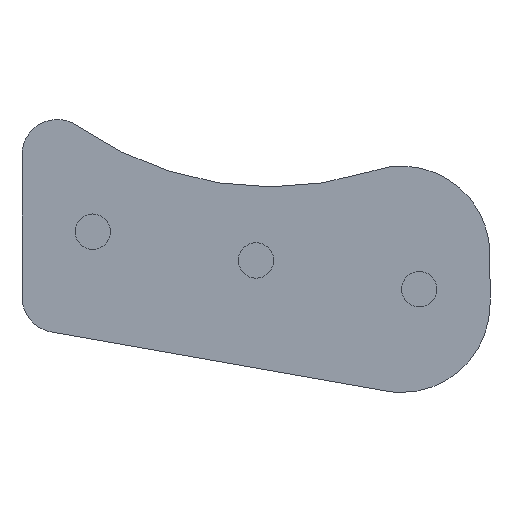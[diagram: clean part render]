
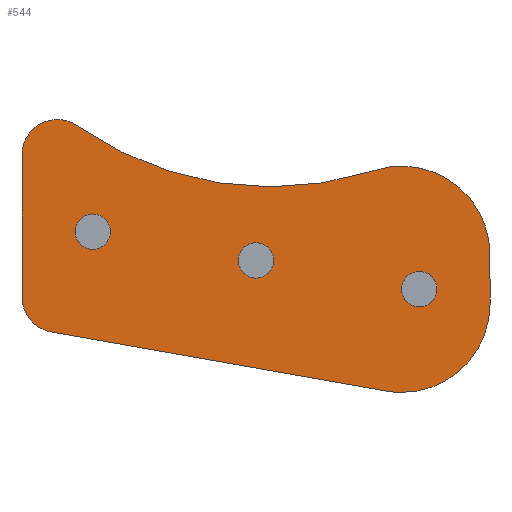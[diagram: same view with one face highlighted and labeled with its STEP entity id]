
A CAD part, left-side view. The second image highlights one B-rep face of the part: STEP entity #544.
In plain terms, the highlighted planar face has unit normal (-1, 0, 0).
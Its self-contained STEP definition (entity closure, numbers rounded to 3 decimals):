
#14 = FACE_BOUND ( 'NONE', #4866, .T. ) ;
#60 = DIRECTION ( 'NONE',  ( 0., 0., -1. ) ) ;
#68 = EDGE_CURVE ( 'NONE', #3412, #212, #5007, .T. ) ;
#90 = CARTESIAN_POINT ( 'NONE',  ( 5., 16.002, -34.415 ) ) ;
#95 = AXIS2_PLACEMENT_3D ( 'NONE', #5192, #797, #5929 ) ;
#101 = DIRECTION ( 'NONE',  ( 0., 0., -1. ) ) ;
#212 = VERTEX_POINT ( 'NONE', #5666 ) ;
#221 = ORIENTED_EDGE ( 'NONE', *, *, #2972, .F. ) ;
#262 = CIRCLE ( 'NONE', #8717, 2.5 ) ;
#370 = ORIENTED_EDGE ( 'NONE', *, *, #1167, .T. ) ;
#393 = DIRECTION ( 'NONE',  ( 1., 0., 0. ) ) ;
#544 = ADVANCED_FACE ( 'NONE', ( #14, #2244, #2038, #2032 ), #2638, .T. ) ;
#551 = CARTESIAN_POINT ( 'NONE',  ( 5., 22.266, -17.584 ) ) ;
#581 = CARTESIAN_POINT ( 'NONE',  ( 5., 8.973, -50.886 ) ) ;
#628 = ORIENTED_EDGE ( 'NONE', *, *, #5931, .T. ) ;
#797 = DIRECTION ( 'NONE',  ( 1., 0., 0. ) ) ;
#824 = DIRECTION ( 'NONE',  ( 0., 0., -1. ) ) ;
#1092 = DIRECTION ( 'NONE',  ( 1., 0., 0. ) ) ;
#1150 = CARTESIAN_POINT ( 'NONE',  ( 5., 16.002, -34.415 ) ) ;
#1167 = EDGE_CURVE ( 'NONE', #2639, #3178, #8629, .T. ) ;
#1358 = CARTESIAN_POINT ( 'NONE',  ( 5., 39.105, -32.842 ) ) ;
#1359 = ORIENTED_EDGE ( 'NONE', *, *, #4983, .F. ) ;
#1401 = VERTEX_POINT ( 'NONE', #3144 ) ;
#1427 = CARTESIAN_POINT ( 'NONE',  ( 5., 16.002, -36.915 ) ) ;
#1443 = ORIENTED_EDGE ( 'NONE', *, *, #1815, .T. ) ;
#1459 = DIRECTION ( 'NONE',  ( 1., 0., 0. ) ) ;
#1531 = VERTEX_POINT ( 'NONE', #3245 ) ;
#1760 = VERTEX_POINT ( 'NONE', #7025 ) ;
#1770 = CARTESIAN_POINT ( 'NONE',  ( 5., 18.502, -36.513 ) ) ;
#1815 = EDGE_CURVE ( 'NONE', #8093, #1892, #6474, .T. ) ;
#1860 = AXIS2_PLACEMENT_3D ( 'NONE', #5502, #1092, #6226 ) ;
#1892 = VERTEX_POINT ( 'NONE', #8812 ) ;
#1895 = DIRECTION ( 'NONE',  ( 0., 0., -1. ) ) ;
#2032 = FACE_OUTER_BOUND ( 'NONE', #8534, .T. ) ;
#2038 = FACE_BOUND ( 'NONE', #4695, .T. ) ;
#2117 = EDGE_CURVE ( 'NONE', #1531, #5927, #5447, .T. ) ;
#2120 = CIRCLE ( 'NONE', #95, 12.5 ) ;
#2172 = CARTESIAN_POINT ( 'NONE',  ( 5., 62.208, -28.768 ) ) ;
#2195 = EDGE_CURVE ( 'NONE', #1760, #6677, #4984, .T. ) ;
#2219 = LINE ( 'NONE', #4430, #2228 ) ;
#2228 = VECTOR ( 'NONE', #60, 1000. ) ;
#2244 = FACE_BOUND ( 'NONE', #3568, .T. ) ;
#2348 = AXIS2_PLACEMENT_3D ( 'NONE', #2391, #7439, #3117 ) ;
#2357 = CARTESIAN_POINT ( 'NONE',  ( 5., 18.502, -29.504 ) ) ;
#2391 = CARTESIAN_POINT ( 'NONE',  ( 5., 62.208, -26.268 ) ) ;
#2432 = EDGE_CURVE ( 'NONE', #4355, #1401, #3818, .T. ) ;
#2502 = DIRECTION ( 'NONE',  ( 0., 0., -1. ) ) ;
#2520 = ORIENTED_EDGE ( 'NONE', *, *, #2117, .T. ) ;
#2608 = ORIENTED_EDGE ( 'NONE', *, *, #68, .F. ) ;
#2638 = PLANE ( 'NONE',  #4228 ) ;
#2639 = VERTEX_POINT ( 'NONE', #5607 ) ;
#2671 = AXIS2_PLACEMENT_3D ( 'NONE', #5453, #1459, #4809 ) ;
#2704 = CARTESIAN_POINT ( 'NONE',  ( 5., 72.208, -15.407 ) ) ;
#2972 = EDGE_CURVE ( 'NONE', #4893, #5985, #2120, .T. ) ;
#3070 = AXIS2_PLACEMENT_3D ( 'NONE', #2357, #7401, #3079 ) ;
#3079 = DIRECTION ( 'NONE',  ( 0., 0., -1. ) ) ;
#3117 = DIRECTION ( 'NONE',  ( 0., 0., -1. ) ) ;
#3144 = CARTESIAN_POINT ( 'NONE',  ( 5., 6.002, -29.504 ) ) ;
#3178 = VERTEX_POINT ( 'NONE', #4520 ) ;
#3245 = CARTESIAN_POINT ( 'NONE',  ( 5., 16.002, -31.915 ) ) ;
#3342 = CARTESIAN_POINT ( 'NONE',  ( 5., 67.208, -35.541 ) ) ;
#3412 = VERTEX_POINT ( 'NONE', #8538 ) ;
#3444 = ORIENTED_EDGE ( 'NONE', *, *, #6522, .T. ) ;
#3568 = EDGE_LOOP ( 'NONE', ( #7085, #2520 ) ) ;
#3595 = DIRECTION ( 'NONE',  ( 1., 0., 0. ) ) ;
#3625 = CARTESIAN_POINT ( 'NONE',  ( 5., 18.502, -49.013 ) ) ;
#3626 = ORIENTED_EDGE ( 'NONE', *, *, #2195, .F. ) ;
#3627 = VECTOR ( 'NONE', #7853, 1000. ) ;
#3639 = CIRCLE ( 'NONE', #2671, 2.5 ) ;
#3818 = CIRCLE ( 'NONE', #3070, 12.5 ) ;
#4075 = DIRECTION ( 'NONE',  ( 0., 0., -1. ) ) ;
#4082 = DIRECTION ( 'NONE',  ( -1., 0., 0. ) ) ;
#4228 = AXIS2_PLACEMENT_3D ( 'NONE', #4833, #4082, #8941 ) ;
#4355 = VERTEX_POINT ( 'NONE', #551 ) ;
#4430 = CARTESIAN_POINT ( 'NONE',  ( 5., 6.002, 0. ) ) ;
#4460 = CIRCLE ( 'NONE', #6195, 5. ) ;
#4476 = CIRCLE ( 'NONE', #8002, 2.5 ) ;
#4479 = DIRECTION ( 'NONE',  ( 1., 0., 0. ) ) ;
#4520 = CARTESIAN_POINT ( 'NONE',  ( 5., 64.335, -11.314 ) ) ;
#4633 = CIRCLE ( 'NONE', #7197, 5. ) ;
#4635 = AXIS2_PLACEMENT_3D ( 'NONE', #90, #5218, #824 ) ;
#4695 = EDGE_LOOP ( 'NONE', ( #3444, #9085 ) ) ;
#4776 = ORIENTED_EDGE ( 'NONE', *, *, #6473, .F. ) ;
#4783 = CARTESIAN_POINT ( 'NONE',  ( 5., 37.042, 27.562 ) ) ;
#4809 = DIRECTION ( 'NONE',  ( 0., 0., -1. ) ) ;
#4833 = CARTESIAN_POINT ( 'NONE',  ( 5., 0., 0. ) ) ;
#4854 = EDGE_CURVE ( 'NONE', #5927, #1531, #4476, .T. ) ;
#4856 = EDGE_CURVE ( 'NONE', #212, #1760, #4460, .T. ) ;
#4866 = EDGE_LOOP ( 'NONE', ( #1443, #628 ) ) ;
#4891 = VECTOR ( 'NONE', #6423, 1000. ) ;
#4893 = VERTEX_POINT ( 'NONE', #5568 ) ;
#4894 = VECTOR ( 'NONE', #7393, 1000. ) ;
#4983 = EDGE_CURVE ( 'NONE', #2639, #4355, #5059, .T. ) ;
#4984 = LINE ( 'NONE', #5284, #4894 ) ;
#5007 = LINE ( 'NONE', #581, #4891 ) ;
#5059 = LINE ( 'NONE', #9109, #3627 ) ;
#5192 = CARTESIAN_POINT ( 'NONE',  ( 5., 18.502, -36.513 ) ) ;
#5218 = DIRECTION ( 'NONE',  ( 1., 0., 0. ) ) ;
#5228 = CIRCLE ( 'NONE', #1860, 2.5 ) ;
#5284 = CARTESIAN_POINT ( 'NONE',  ( 5., 72.208, 0. ) ) ;
#5447 = CIRCLE ( 'NONE', #4635, 2.5 ) ;
#5453 = CARTESIAN_POINT ( 'NONE',  ( 5., 39.105, -30.342 ) ) ;
#5502 = CARTESIAN_POINT ( 'NONE',  ( 5., 39.105, -30.342 ) ) ;
#5519 = DIRECTION ( 'NONE',  ( 0., 0., -1. ) ) ;
#5568 = CARTESIAN_POINT ( 'NONE',  ( 5., 6.002, -36.513 ) ) ;
#5607 = CARTESIAN_POINT ( 'NONE',  ( 5., 22.739, -17.734 ) ) ;
#5666 = CARTESIAN_POINT ( 'NONE',  ( 5., 68.076, -40.465 ) ) ;
#5680 = CIRCLE ( 'NONE', #9104, 12.5 ) ;
#5902 = ORIENTED_EDGE ( 'NONE', *, *, #2432, .F. ) ;
#5927 = VERTEX_POINT ( 'NONE', #1427 ) ;
#5929 = DIRECTION ( 'NONE',  ( 0., 0., -1. ) ) ;
#5931 = EDGE_CURVE ( 'NONE', #1892, #8093, #262, .T. ) ;
#5984 = CARTESIAN_POINT ( 'NONE',  ( 5., 39.105, -27.842 ) ) ;
#5985 = VERTEX_POINT ( 'NONE', #3625 ) ;
#6195 = AXIS2_PLACEMENT_3D ( 'NONE', #3342, #8302, #4075 ) ;
#6226 = DIRECTION ( 'NONE',  ( 0., 0., -1. ) ) ;
#6285 = DIRECTION ( 'NONE',  ( 1., 0., 0. ) ) ;
#6423 = DIRECTION ( 'NONE',  ( 0., 0.985, 0.174 ) ) ;
#6473 = EDGE_CURVE ( 'NONE', #5985, #3412, #5680, .T. ) ;
#6474 = CIRCLE ( 'NONE', #2348, 2.5 ) ;
#6522 = EDGE_CURVE ( 'NONE', #7081, #7227, #5228, .T. ) ;
#6531 = ORIENTED_EDGE ( 'NONE', *, *, #4856, .F. ) ;
#6677 = VERTEX_POINT ( 'NONE', #2704 ) ;
#6830 = EDGE_CURVE ( 'NONE', #6677, #3178, #4633, .T. ) ;
#6844 = DIRECTION ( 'NONE',  ( 1., 0., 0. ) ) ;
#6933 = EDGE_CURVE ( 'NONE', #7227, #7081, #3639, .T. ) ;
#7008 = ORIENTED_EDGE ( 'NONE', *, *, #6830, .F. ) ;
#7025 = CARTESIAN_POINT ( 'NONE',  ( 5., 72.208, -35.541 ) ) ;
#7081 = VERTEX_POINT ( 'NONE', #1358 ) ;
#7085 = ORIENTED_EDGE ( 'NONE', *, *, #4854, .T. ) ;
#7155 = EDGE_CURVE ( 'NONE', #1401, #4893, #2219, .T. ) ;
#7197 = AXIS2_PLACEMENT_3D ( 'NONE', #8626, #4479, #101 ) ;
#7227 = VERTEX_POINT ( 'NONE', #5984 ) ;
#7245 = AXIS2_PLACEMENT_3D ( 'NONE', #4783, #393, #5519 ) ;
#7393 = DIRECTION ( 'NONE',  ( 0., 0., 1. ) ) ;
#7401 = DIRECTION ( 'NONE',  ( 1., 0., 0. ) ) ;
#7439 = DIRECTION ( 'NONE',  ( 1., 0., 0. ) ) ;
#7853 = DIRECTION ( 'NONE',  ( 0., -0.954, 0.301 ) ) ;
#7900 = CARTESIAN_POINT ( 'NONE',  ( 5., 62.208, -26.268 ) ) ;
#8002 = AXIS2_PLACEMENT_3D ( 'NONE', #1150, #6285, #1895 ) ;
#8093 = VERTEX_POINT ( 'NONE', #2172 ) ;
#8302 = DIRECTION ( 'NONE',  ( 1., 0., 0. ) ) ;
#8534 = EDGE_LOOP ( 'NONE', ( #3626, #6531, #2608, #4776, #221, #8669, #5902, #1359, #370, #7008 ) ) ;
#8538 = CARTESIAN_POINT ( 'NONE',  ( 5., 20.673, -48.823 ) ) ;
#8549 = DIRECTION ( 'NONE',  ( 0., 0., -1. ) ) ;
#8626 = CARTESIAN_POINT ( 'NONE',  ( 5., 67.208, -15.407 ) ) ;
#8629 = CIRCLE ( 'NONE', #7245, 47.5 ) ;
#8669 = ORIENTED_EDGE ( 'NONE', *, *, #7155, .F. ) ;
#8717 = AXIS2_PLACEMENT_3D ( 'NONE', #7900, #3595, #8549 ) ;
#8812 = CARTESIAN_POINT ( 'NONE',  ( 5., 62.208, -23.768 ) ) ;
#8941 = DIRECTION ( 'NONE',  ( 0., 0., -1. ) ) ;
#9085 = ORIENTED_EDGE ( 'NONE', *, *, #6933, .T. ) ;
#9104 = AXIS2_PLACEMENT_3D ( 'NONE', #1770, #6844, #2502 ) ;
#9109 = CARTESIAN_POINT ( 'NONE',  ( 5., -3.03, -9.596 ) ) ;
